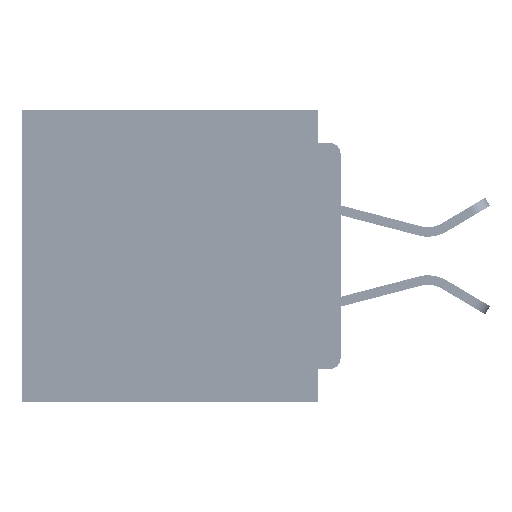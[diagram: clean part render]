
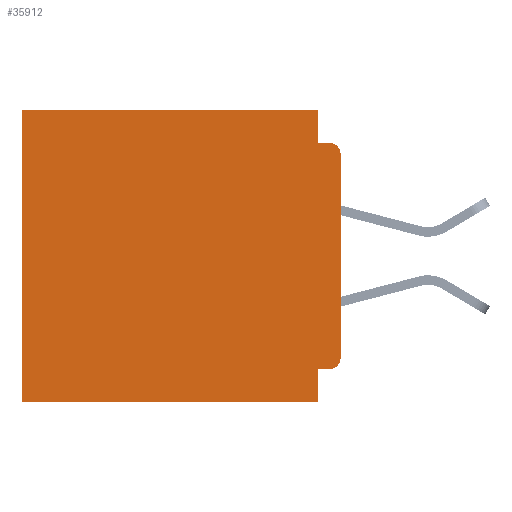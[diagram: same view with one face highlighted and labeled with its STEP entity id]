
A CAD part, left-side view. The second image highlights one B-rep face of the part: STEP entity #35912.
In plain terms, the highlighted planar face has unit normal (-1, 0, 0).
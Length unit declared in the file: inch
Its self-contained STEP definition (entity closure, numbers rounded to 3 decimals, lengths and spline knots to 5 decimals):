
#655 = VECTOR ( 'NONE', #11760, 39.37008 ) ;
#1183 = CARTESIAN_POINT ( 'NONE',  ( 0.3, 0.031, -0.355 ) ) ;
#3287 = CARTESIAN_POINT ( 'NONE',  ( 0.3, 0., -0.4 ) ) ;
#3634 = DIRECTION ( 'NONE',  ( 0., 0., -1. ) ) ;
#4077 = ORIENTED_EDGE ( 'NONE', *, *, #57064, .F. ) ;
#4123 = LINE ( 'NONE', #29601, #25106 ) ;
#4771 = CARTESIAN_POINT ( 'NONE',  ( 0.3, 0.031, 0. ) ) ;
#5843 = AXIS2_PLACEMENT_3D ( 'NONE', #56799, #30329, #3634 ) ;
#5892 = VECTOR ( 'NONE', #7800, 39.37008 ) ;
#6388 = DIRECTION ( 'NONE',  ( 0., 0., -1. ) ) ;
#6510 = VECTOR ( 'NONE', #6388, 39.37008 ) ;
#6878 = CARTESIAN_POINT ( 'NONE',  ( 0.3, 0., -0.045 ) ) ;
#7268 = VECTOR ( 'NONE', #10339, 39.37008 ) ;
#7406 = PLANE ( 'NONE',  #9424 ) ;
#7618 = ORIENTED_EDGE ( 'NONE', *, *, #54121, .F. ) ;
#7800 = DIRECTION ( 'NONE',  ( 0., 1., 0. ) ) ;
#8058 = CARTESIAN_POINT ( 'NONE',  ( 0.3, 0., -0.4 ) ) ;
#8709 = CARTESIAN_POINT ( 'NONE',  ( 0.3, 0.437, -0.4 ) ) ;
#9424 = AXIS2_PLACEMENT_3D ( 'NONE', #11871, #25376, #56280 ) ;
#9683 = EDGE_CURVE ( 'NONE', #27928, #20808, #25033, .T. ) ;
#10339 = DIRECTION ( 'NONE',  ( 0., 1., 0. ) ) ;
#10536 = CARTESIAN_POINT ( 'NONE',  ( 0.3, 0., -0.34 ) ) ;
#11666 = DIRECTION ( 'NONE',  ( 0., 1., 0. ) ) ;
#11691 = VERTEX_POINT ( 'NONE', #26179 ) ;
#11760 = DIRECTION ( 'NONE',  ( 0., 0., -1. ) ) ;
#11871 = CARTESIAN_POINT ( 'NONE',  ( 0.3, 0., -0.4 ) ) ;
#11879 = EDGE_CURVE ( 'NONE', #32098, #14339, #17667, .T. ) ;
#12450 = ORIENTED_EDGE ( 'NONE', *, *, #29807, .T. ) ;
#12469 = LINE ( 'NONE', #25079, #655 ) ;
#12594 = LINE ( 'NONE', #8058, #34834 ) ;
#14339 = VERTEX_POINT ( 'NONE', #10536 ) ;
#15323 = CARTESIAN_POINT ( 'NONE',  ( 0.3, 0.031, -0.4 ) ) ;
#15456 = ORIENTED_EDGE ( 'NONE', *, *, #35367, .F. ) ;
#16220 = EDGE_CURVE ( 'NONE', #48435, #32802, #22445, .T. ) ;
#17667 = CIRCLE ( 'NONE', #38525, 0.015 ) ;
#18286 = ORIENTED_EDGE ( 'NONE', *, *, #16220, .T. ) ;
#19760 = CARTESIAN_POINT ( 'NONE',  ( 0.3, 0.015, -0.34 ) ) ;
#20808 = VERTEX_POINT ( 'NONE', #55051 ) ;
#22445 = LINE ( 'NONE', #43113, #44549 ) ;
#24281 = DIRECTION ( 'NONE',  ( 0., 0., -1. ) ) ;
#25033 = LINE ( 'NONE', #6878, #51341 ) ;
#25079 = CARTESIAN_POINT ( 'NONE',  ( 0.3, 0.031, 0. ) ) ;
#25106 = VECTOR ( 'NONE', #11666, 39.37008 ) ;
#25376 = DIRECTION ( 'NONE',  ( 1., 0., 0. ) ) ;
#26179 = CARTESIAN_POINT ( 'NONE',  ( 0.3, 0.031, -0.4 ) ) ;
#26575 = CARTESIAN_POINT ( 'NONE',  ( 0.3, 0.437, 0. ) ) ;
#27348 = CIRCLE ( 'NONE', #5843, 0.015 ) ;
#27928 = VERTEX_POINT ( 'NONE', #31928 ) ;
#28209 = LINE ( 'NONE', #3287, #5892 ) ;
#29601 = CARTESIAN_POINT ( 'NONE',  ( 0.3, 0., 0. ) ) ;
#29807 = EDGE_CURVE ( 'NONE', #44763, #20808, #27348, .T. ) ;
#30182 = LINE ( 'NONE', #15323, #6510 ) ;
#30329 = DIRECTION ( 'NONE',  ( -1., 0., 0. ) ) ;
#31928 = CARTESIAN_POINT ( 'NONE',  ( 0.3, 0.031, -0.045 ) ) ;
#32083 = EDGE_CURVE ( 'NONE', #36699, #48435, #4123, .T. ) ;
#32098 = VERTEX_POINT ( 'NONE', #47373 ) ;
#32802 = VERTEX_POINT ( 'NONE', #8709 ) ;
#33513 = DIRECTION ( 'NONE',  ( 0., -1., 0. ) ) ;
#34212 = DIRECTION ( 'NONE',  ( 0., 0., -1. ) ) ;
#34625 = ORIENTED_EDGE ( 'NONE', *, *, #32083, .T. ) ;
#34663 = DIRECTION ( 'NONE',  ( 0., 0., -1. ) ) ;
#34834 = VECTOR ( 'NONE', #34663, 39.37008 ) ;
#35367 = EDGE_CURVE ( 'NONE', #44763, #14339, #12594, .T. ) ;
#35782 = EDGE_LOOP ( 'NONE', ( #15456, #12450, #54304, #4077, #34625, #18286, #42456, #7618, #49943, #37829 ) ) ;
#35912 = ADVANCED_FACE ( 'NONE', ( #42401 ), #7406, .F. ) ;
#36699 = VERTEX_POINT ( 'NONE', #4771 ) ;
#37829 = ORIENTED_EDGE ( 'NONE', *, *, #11879, .T. ) ;
#38525 = AXIS2_PLACEMENT_3D ( 'NONE', #19760, #50777, #24281 ) ;
#42401 = FACE_OUTER_BOUND ( 'NONE', #35782, .T. ) ;
#42456 = ORIENTED_EDGE ( 'NONE', *, *, #48950, .F. ) ;
#42931 = VERTEX_POINT ( 'NONE', #1183 ) ;
#43113 = CARTESIAN_POINT ( 'NONE',  ( 0.3, 0.437, -0.4 ) ) ;
#44549 = VECTOR ( 'NONE', #34212, 39.37008 ) ;
#44763 = VERTEX_POINT ( 'NONE', #46756 ) ;
#46033 = CARTESIAN_POINT ( 'NONE',  ( 0.3, 0., -0.355 ) ) ;
#46756 = CARTESIAN_POINT ( 'NONE',  ( 0.3, 0., -0.06 ) ) ;
#47373 = CARTESIAN_POINT ( 'NONE',  ( 0.3, 0.015, -0.355 ) ) ;
#48435 = VERTEX_POINT ( 'NONE', #26575 ) ;
#48950 = EDGE_CURVE ( 'NONE', #11691, #32802, #28209, .T. ) ;
#49943 = ORIENTED_EDGE ( 'NONE', *, *, #53534, .F. ) ;
#50777 = DIRECTION ( 'NONE',  ( -1., 0., 0. ) ) ;
#51341 = VECTOR ( 'NONE', #33513, 39.37008 ) ;
#53112 = LINE ( 'NONE', #46033, #7268 ) ;
#53534 = EDGE_CURVE ( 'NONE', #32098, #42931, #53112, .T. ) ;
#54121 = EDGE_CURVE ( 'NONE', #42931, #11691, #30182, .T. ) ;
#54304 = ORIENTED_EDGE ( 'NONE', *, *, #9683, .F. ) ;
#55051 = CARTESIAN_POINT ( 'NONE',  ( 0.3, 0.015, -0.045 ) ) ;
#56280 = DIRECTION ( 'NONE',  ( 0., 0., -1. ) ) ;
#56799 = CARTESIAN_POINT ( 'NONE',  ( 0.3, 0.015, -0.06 ) ) ;
#57064 = EDGE_CURVE ( 'NONE', #36699, #27928, #12469, .T. ) ;
